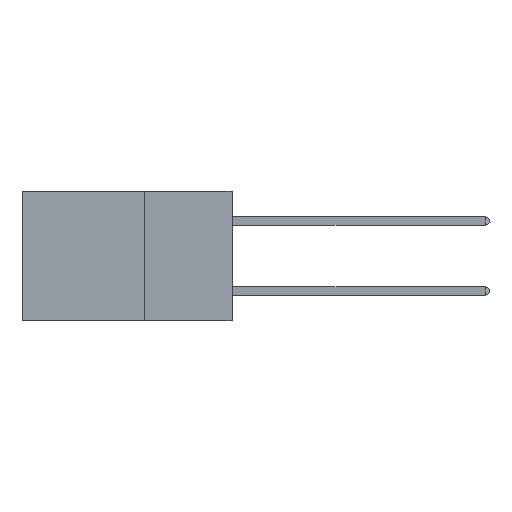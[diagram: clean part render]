
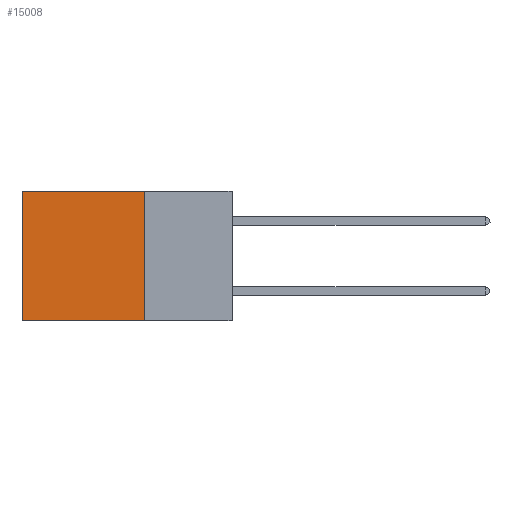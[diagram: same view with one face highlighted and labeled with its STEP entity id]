
A CAD part, left-side view. The second image highlights one B-rep face of the part: STEP entity #15008.
In plain terms, the highlighted planar face has unit normal (-1, 0, 0).
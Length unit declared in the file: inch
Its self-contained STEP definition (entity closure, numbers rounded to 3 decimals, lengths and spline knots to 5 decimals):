
#436 = EDGE_CURVE ( 'NONE', #11100, #15335, #1989, .T. ) ;
#1137 = VERTEX_POINT ( 'NONE', #3229 ) ;
#1622 = DIRECTION ( 'NONE',  ( 0., 0., -1. ) ) ;
#1989 = LINE ( 'NONE', #16808, #16202 ) ;
#2121 = LINE ( 'NONE', #5197, #10312 ) ;
#2438 = DIRECTION ( 'NONE',  ( 0., 1., 0. ) ) ;
#3229 = CARTESIAN_POINT ( 'NONE',  ( 0.2875, 0.25, -0.37 ) ) ;
#3383 = EDGE_CURVE ( 'NONE', #11100, #1137, #2121, .T. ) ;
#3465 = AXIS2_PLACEMENT_3D ( 'NONE', #11289, #12646, #3529 ) ;
#3529 = DIRECTION ( 'NONE',  ( 0., 0., -1. ) ) ;
#3598 = ORIENTED_EDGE ( 'NONE', *, *, #11338, .T. ) ;
#4191 = ORIENTED_EDGE ( 'NONE', *, *, #436, .T. ) ;
#4614 = CARTESIAN_POINT ( 'NONE',  ( 0.2875, 0.6, -0.37 ) ) ;
#5121 = EDGE_LOOP ( 'NONE', ( #3598, #7142, #14225, #4191 ) ) ;
#5197 = CARTESIAN_POINT ( 'NONE',  ( 0.2875, 0.25, 0. ) ) ;
#5363 = CARTESIAN_POINT ( 'NONE',  ( 0.2875, 0.25, 0. ) ) ;
#6208 = VECTOR ( 'NONE', #15175, 39.37008 ) ;
#6566 = DIRECTION ( 'NONE',  ( 0., 1., 0. ) ) ;
#7142 = ORIENTED_EDGE ( 'NONE', *, *, #16336, .F. ) ;
#8008 = CARTESIAN_POINT ( 'NONE',  ( 0.2875, 0.6, 0. ) ) ;
#8172 = LINE ( 'NONE', #14171, #11936 ) ;
#8877 = VERTEX_POINT ( 'NONE', #4614 ) ;
#10037 = CARTESIAN_POINT ( 'NONE',  ( 0.2875, 0.6, 0. ) ) ;
#10312 = VECTOR ( 'NONE', #1622, 39.37008 ) ;
#11100 = VERTEX_POINT ( 'NONE', #5363 ) ;
#11289 = CARTESIAN_POINT ( 'NONE',  ( 0.2875, 0.25, 0. ) ) ;
#11338 = EDGE_CURVE ( 'NONE', #15335, #8877, #16894, .T. ) ;
#11586 = FACE_OUTER_BOUND ( 'NONE', #5121, .T. ) ;
#11936 = VECTOR ( 'NONE', #2438, 39.37008 ) ;
#12646 = DIRECTION ( 'NONE',  ( 1., 0., 0. ) ) ;
#14171 = CARTESIAN_POINT ( 'NONE',  ( 0.2875, 0.25, -0.37 ) ) ;
#14225 = ORIENTED_EDGE ( 'NONE', *, *, #3383, .F. ) ;
#15008 = ADVANCED_FACE ( 'NONE', ( #11586 ), #15203, .F. ) ;
#15175 = DIRECTION ( 'NONE',  ( 0., 0., -1. ) ) ;
#15203 = PLANE ( 'NONE',  #3465 ) ;
#15335 = VERTEX_POINT ( 'NONE', #8008 ) ;
#16202 = VECTOR ( 'NONE', #6566, 39.37008 ) ;
#16336 = EDGE_CURVE ( 'NONE', #1137, #8877, #8172, .T. ) ;
#16808 = CARTESIAN_POINT ( 'NONE',  ( 0.2875, 0.25, 0. ) ) ;
#16894 = LINE ( 'NONE', #10037, #6208 ) ;
